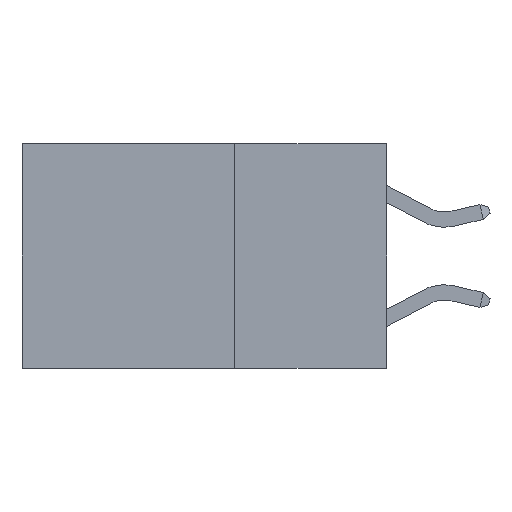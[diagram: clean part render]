
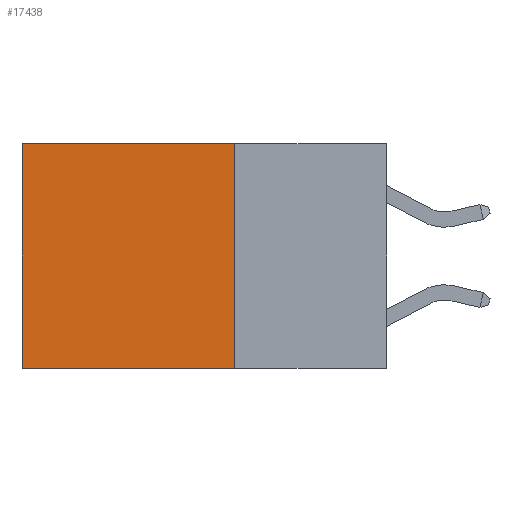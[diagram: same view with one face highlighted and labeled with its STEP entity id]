
A CAD part, left-side view. The second image highlights one B-rep face of the part: STEP entity #17438.
In plain terms, the highlighted planar face has unit normal (-1, 0, 0).
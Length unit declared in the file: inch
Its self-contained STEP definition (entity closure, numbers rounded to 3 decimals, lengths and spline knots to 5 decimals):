
#244 = DIRECTION ( 'NONE',  ( 0., 0., -1. ) ) ;
#760 = CARTESIAN_POINT ( 'NONE',  ( 0.2625, 0.25, 0. ) ) ;
#1188 = CARTESIAN_POINT ( 'NONE',  ( 0.2625, 0.25, 0. ) ) ;
#1816 = VECTOR ( 'NONE', #17983, 39.37008 ) ;
#2070 = CARTESIAN_POINT ( 'NONE',  ( 0.2625, 0.25, 0. ) ) ;
#3728 = EDGE_CURVE ( 'NONE', #10491, #27245, #16400, .T. ) ;
#4615 = PLANE ( 'NONE',  #10988 ) ;
#4882 = EDGE_LOOP ( 'NONE', ( #22443, #8135, #9134, #13515 ) ) ;
#6257 = VECTOR ( 'NONE', #9936, 39.37008 ) ;
#8135 = ORIENTED_EDGE ( 'NONE', *, *, #16048, .F. ) ;
#8372 = CARTESIAN_POINT ( 'NONE',  ( 0.2625, 0.25, -0.37 ) ) ;
#9134 = ORIENTED_EDGE ( 'NONE', *, *, #19191, .F. ) ;
#9663 = VERTEX_POINT ( 'NONE', #8372 ) ;
#9936 = DIRECTION ( 'NONE',  ( 0., 1., 0. ) ) ;
#10491 = VERTEX_POINT ( 'NONE', #17908 ) ;
#10988 = AXIS2_PLACEMENT_3D ( 'NONE', #2070, #23097, #29527 ) ;
#13498 = FACE_OUTER_BOUND ( 'NONE', #4882, .T. ) ;
#13515 = ORIENTED_EDGE ( 'NONE', *, *, #21603, .T. ) ;
#13733 = DIRECTION ( 'NONE',  ( 0., 0., -1. ) ) ;
#16048 = EDGE_CURVE ( 'NONE', #9663, #27245, #22509, .T. ) ;
#16400 = LINE ( 'NONE', #25560, #27669 ) ;
#16543 = LINE ( 'NONE', #760, #6257 ) ;
#17438 = ADVANCED_FACE ( 'NONE', ( #13498 ), #4615, .F. ) ;
#17908 = CARTESIAN_POINT ( 'NONE',  ( 0.2625, 0.6, 0. ) ) ;
#17983 = DIRECTION ( 'NONE',  ( 0., 1., 0. ) ) ;
#18429 = CARTESIAN_POINT ( 'NONE',  ( 0.2625, 0.25, 0. ) ) ;
#18580 = CARTESIAN_POINT ( 'NONE',  ( 0.2625, 0.6, -0.37 ) ) ;
#19191 = EDGE_CURVE ( 'NONE', #23862, #9663, #27143, .T. ) ;
#20257 = CARTESIAN_POINT ( 'NONE',  ( 0.2625, 0.25, -0.37 ) ) ;
#21603 = EDGE_CURVE ( 'NONE', #23862, #10491, #16543, .T. ) ;
#22087 = VECTOR ( 'NONE', #244, 39.37008 ) ;
#22443 = ORIENTED_EDGE ( 'NONE', *, *, #3728, .T. ) ;
#22509 = LINE ( 'NONE', #20257, #1816 ) ;
#23097 = DIRECTION ( 'NONE',  ( 1., 0., 0. ) ) ;
#23862 = VERTEX_POINT ( 'NONE', #1188 ) ;
#25560 = CARTESIAN_POINT ( 'NONE',  ( 0.2625, 0.6, 0. ) ) ;
#27143 = LINE ( 'NONE', #18429, #22087 ) ;
#27245 = VERTEX_POINT ( 'NONE', #18580 ) ;
#27669 = VECTOR ( 'NONE', #13733, 39.37008 ) ;
#29527 = DIRECTION ( 'NONE',  ( 0., 0., -1. ) ) ;
